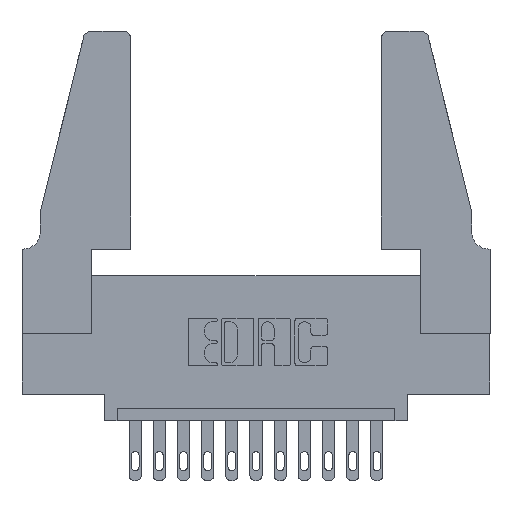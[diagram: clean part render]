
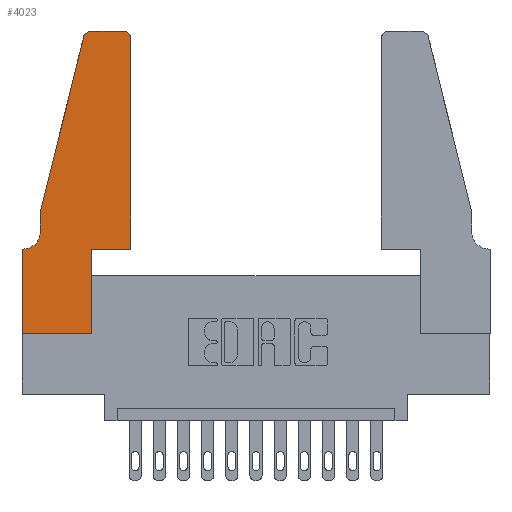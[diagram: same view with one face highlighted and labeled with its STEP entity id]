
A CAD part, top view. The second image highlights one B-rep face of the part: STEP entity #4023.
In plain terms, the highlighted planar face has unit normal (0, 0, 1).
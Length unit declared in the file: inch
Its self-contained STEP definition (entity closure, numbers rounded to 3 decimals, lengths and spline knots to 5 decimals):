
#29 = EDGE_CURVE ( 'NONE', #7411, #5335, #12930, .T. ) ;
#95 = VECTOR ( 'NONE', #14174, 39.37008 ) ;
#540 = LINE ( 'NONE', #13804, #9423 ) ;
#749 = AXIS2_PLACEMENT_3D ( 'NONE', #7501, #10041, #11949 ) ;
#812 = CARTESIAN_POINT ( 'NONE',  ( 0.284, 1.25, 0.37 ) ) ;
#822 = LINE ( 'NONE', #6305, #7931 ) ;
#1032 = ORIENTED_EDGE ( 'NONE', *, *, #9598, .T. ) ;
#1095 = VECTOR ( 'NONE', #14602, 39.37008 ) ;
#1167 = LINE ( 'NONE', #8537, #95 ) ;
#1207 = DIRECTION ( 'NONE',  ( 0., 1., 0. ) ) ;
#1235 = CIRCLE ( 'NONE', #12239, 0.03 ) ;
#1553 = VECTOR ( 'NONE', #3323, 39.37008 ) ;
#1737 = LINE ( 'NONE', #14426, #5132 ) ;
#1755 = LINE ( 'NONE', #10933, #11330 ) ;
#1777 = EDGE_CURVE ( 'NONE', #5335, #4407, #822, .T. ) ;
#1935 = VERTEX_POINT ( 'NONE', #3499 ) ;
#2130 = VERTEX_POINT ( 'NONE', #6979 ) ;
#2299 = VERTEX_POINT ( 'NONE', #812 ) ;
#2676 = ORIENTED_EDGE ( 'NONE', *, *, #4410, .T. ) ;
#2783 = EDGE_CURVE ( 'NONE', #11799, #5987, #8594, .T. ) ;
#2827 = DIRECTION ( 'NONE',  ( 1., 0., 0. ) ) ;
#2918 = CARTESIAN_POINT ( 'NONE',  ( 0.0055, 0.35, 0.37 ) ) ;
#3010 = CIRCLE ( 'NONE', #11484, 0.07 ) ;
#3323 = DIRECTION ( 'NONE',  ( 0., -1., 0. ) ) ;
#3378 = CARTESIAN_POINT ( 'NONE',  ( 0., 0., 0.37 ) ) ;
#3499 = CARTESIAN_POINT ( 'NONE',  ( 0.25487, 1.22718, 0.37 ) ) ;
#3725 = CARTESIAN_POINT ( 'NONE',  ( 0.0755, 0.42, 0.37 ) ) ;
#3761 = CARTESIAN_POINT ( 'NONE',  ( 0., 0.35, 0.37 ) ) ;
#4023 = ADVANCED_FACE ( 'NONE', ( #8390 ), #12968, .T. ) ;
#4201 = ORIENTED_EDGE ( 'NONE', *, *, #6652, .T. ) ;
#4222 = CARTESIAN_POINT ( 'NONE',  ( 0.0055, 0.42, 0.37 ) ) ;
#4407 = VERTEX_POINT ( 'NONE', #5440 ) ;
#4410 = EDGE_CURVE ( 'NONE', #5422, #2299, #14383, .T. ) ;
#4453 = CARTESIAN_POINT ( 'NONE',  ( 0.2605, 1.25, 0.37 ) ) ;
#5049 = VERTEX_POINT ( 'NONE', #13431 ) ;
#5132 = VECTOR ( 'NONE', #5348, 39.37008 ) ;
#5335 = VERTEX_POINT ( 'NONE', #11027 ) ;
#5348 = DIRECTION ( 'NONE',  ( 0., 1., 0. ) ) ;
#5389 = AXIS2_PLACEMENT_3D ( 'NONE', #3761, #10354, #12675 ) ;
#5411 = ORIENTED_EDGE ( 'NONE', *, *, #8564, .T. ) ;
#5422 = VERTEX_POINT ( 'NONE', #14354 ) ;
#5440 = CARTESIAN_POINT ( 'NONE',  ( 0.2865, 0., 0.37 ) ) ;
#5515 = EDGE_LOOP ( 'NONE', ( #2676, #9315, #1032, #9189, #11080, #4201, #12276, #11028, #12753, #12094, #10231, #5411 ) ) ;
#5677 = CIRCLE ( 'NONE', #749, 0.03 ) ;
#5909 = EDGE_CURVE ( 'NONE', #2299, #1935, #1235, .T. ) ;
#5987 = VERTEX_POINT ( 'NONE', #3725 ) ;
#6162 = CARTESIAN_POINT ( 'NONE',  ( 0.284, 1.22, 0.37 ) ) ;
#6305 = CARTESIAN_POINT ( 'NONE',  ( 0., 0., 0.37 ) ) ;
#6626 = CARTESIAN_POINT ( 'NONE',  ( 0.0755, 0.5, 0.37 ) ) ;
#6652 = EDGE_CURVE ( 'NONE', #12462, #7411, #1755, .T. ) ;
#6667 = DIRECTION ( 'NONE',  ( 0., -1., 0. ) ) ;
#6869 = EDGE_CURVE ( 'NONE', #13563, #5049, #1737, .T. ) ;
#6979 = CARTESIAN_POINT ( 'NONE',  ( 0.2865, 0.35, 0.37 ) ) ;
#7275 = DIRECTION ( 'NONE',  ( 0., 0., 1. ) ) ;
#7411 = VERTEX_POINT ( 'NONE', #13164 ) ;
#7501 = CARTESIAN_POINT ( 'NONE',  ( 0.4205, 1.22, 0.37 ) ) ;
#7931 = VECTOR ( 'NONE', #2827, 39.37008 ) ;
#8372 = EDGE_CURVE ( 'NONE', #5987, #12462, #3010, .T. ) ;
#8390 = FACE_OUTER_BOUND ( 'NONE', #5515, .T. ) ;
#8537 = CARTESIAN_POINT ( 'NONE',  ( 0.0755, 0.5, 0.37 ) ) ;
#8564 = EDGE_CURVE ( 'NONE', #5049, #5422, #5677, .T. ) ;
#8594 = LINE ( 'NONE', #6626, #8784 ) ;
#8784 = VECTOR ( 'NONE', #6667, 39.37008 ) ;
#9147 = CARTESIAN_POINT ( 'NONE',  ( 0.2865, 0.35, 0.37 ) ) ;
#9189 = ORIENTED_EDGE ( 'NONE', *, *, #2783, .T. ) ;
#9315 = ORIENTED_EDGE ( 'NONE', *, *, #5909, .T. ) ;
#9423 = VECTOR ( 'NONE', #13889, 39.37008 ) ;
#9598 = EDGE_CURVE ( 'NONE', #1935, #11799, #1167, .T. ) ;
#9657 = DIRECTION ( 'NONE',  ( 1., 0., 0. ) ) ;
#10041 = DIRECTION ( 'NONE',  ( 0., 0., 1. ) ) ;
#10231 = ORIENTED_EDGE ( 'NONE', *, *, #6869, .T. ) ;
#10354 = DIRECTION ( 'NONE',  ( 0., 0., 1. ) ) ;
#10722 = LINE ( 'NONE', #9147, #11227 ) ;
#10920 = DIRECTION ( 'NONE',  ( 0., 0., -1. ) ) ;
#10933 = CARTESIAN_POINT ( 'NONE',  ( 0.0755, 0.35, 0.37 ) ) ;
#11027 = CARTESIAN_POINT ( 'NONE',  ( 0., 0., 0.37 ) ) ;
#11028 = ORIENTED_EDGE ( 'NONE', *, *, #1777, .T. ) ;
#11080 = ORIENTED_EDGE ( 'NONE', *, *, #8372, .T. ) ;
#11227 = VECTOR ( 'NONE', #1207, 39.37008 ) ;
#11330 = VECTOR ( 'NONE', #13286, 39.37008 ) ;
#11484 = AXIS2_PLACEMENT_3D ( 'NONE', #4222, #10920, #12142 ) ;
#11799 = VERTEX_POINT ( 'NONE', #13066 ) ;
#11949 = DIRECTION ( 'NONE',  ( 1., 0., 0. ) ) ;
#12094 = ORIENTED_EDGE ( 'NONE', *, *, #13477, .T. ) ;
#12142 = DIRECTION ( 'NONE',  ( -1., 0., 0. ) ) ;
#12239 = AXIS2_PLACEMENT_3D ( 'NONE', #6162, #7275, #9657 ) ;
#12276 = ORIENTED_EDGE ( 'NONE', *, *, #29, .T. ) ;
#12462 = VERTEX_POINT ( 'NONE', #2918 ) ;
#12675 = DIRECTION ( 'NONE',  ( 1., 0., 0. ) ) ;
#12753 = ORIENTED_EDGE ( 'NONE', *, *, #13915, .T. ) ;
#12930 = LINE ( 'NONE', #3378, #1553 ) ;
#12968 = PLANE ( 'NONE',  #5389 ) ;
#13066 = CARTESIAN_POINT ( 'NONE',  ( 0.0755, 0.5, 0.37 ) ) ;
#13164 = CARTESIAN_POINT ( 'NONE',  ( 0., 0.35, 0.37 ) ) ;
#13286 = DIRECTION ( 'NONE',  ( -1., 0., 0. ) ) ;
#13431 = CARTESIAN_POINT ( 'NONE',  ( 0.4505, 1.22, 0.37 ) ) ;
#13477 = EDGE_CURVE ( 'NONE', #2130, #13563, #540, .T. ) ;
#13563 = VERTEX_POINT ( 'NONE', #14280 ) ;
#13804 = CARTESIAN_POINT ( 'NONE',  ( 0.4505, 0.35, 0.37 ) ) ;
#13889 = DIRECTION ( 'NONE',  ( 1., 0., 0. ) ) ;
#13915 = EDGE_CURVE ( 'NONE', #4407, #2130, #10722, .T. ) ;
#14174 = DIRECTION ( 'NONE',  ( -0.239, -0.971, 0. ) ) ;
#14280 = CARTESIAN_POINT ( 'NONE',  ( 0.4505, 0.35, 0.37 ) ) ;
#14354 = CARTESIAN_POINT ( 'NONE',  ( 0.4205, 1.25, 0.37 ) ) ;
#14383 = LINE ( 'NONE', #4453, #1095 ) ;
#14426 = CARTESIAN_POINT ( 'NONE',  ( 0.4505, 0.35, 0.37 ) ) ;
#14602 = DIRECTION ( 'NONE',  ( -1., 0., 0. ) ) ;
